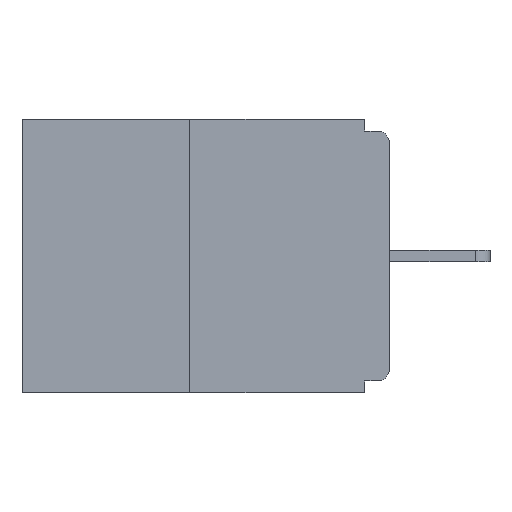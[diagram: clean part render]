
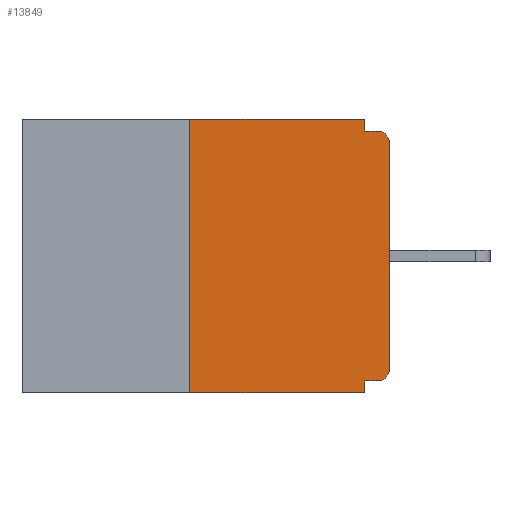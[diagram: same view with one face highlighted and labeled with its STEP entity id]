
A CAD part, left-side view. The second image highlights one B-rep face of the part: STEP entity #13849.
In plain terms, the highlighted planar face has unit normal (-1, 0, 0).
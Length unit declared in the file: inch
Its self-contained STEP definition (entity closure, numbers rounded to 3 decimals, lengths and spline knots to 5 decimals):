
#448 = DIRECTION ( 'NONE',  ( 0., -1., 0. ) ) ;
#521 = VECTOR ( 'NONE', #5096, 39.37008 ) ;
#563 = LINE ( 'NONE', #6883, #10628 ) ;
#835 = DIRECTION ( 'NONE',  ( 0., 0., -1. ) ) ;
#1184 = LINE ( 'NONE', #11006, #7545 ) ;
#1287 = DIRECTION ( 'NONE',  ( 0., -1., 0. ) ) ;
#1321 = VECTOR ( 'NONE', #2225, 39.37008 ) ;
#1588 = CARTESIAN_POINT ( 'NONE',  ( 0., 0.25, 0. ) ) ;
#1994 = CARTESIAN_POINT ( 'NONE',  ( 0., 0.031, 0. ) ) ;
#2058 = ORIENTED_EDGE ( 'NONE', *, *, #6937, .F. ) ;
#2107 = EDGE_CURVE ( 'NONE', #11901, #16938, #563, .T. ) ;
#2209 = ORIENTED_EDGE ( 'NONE', *, *, #16745, .F. ) ;
#2225 = DIRECTION ( 'NONE',  ( 0., 0., 1. ) ) ;
#2241 = CARTESIAN_POINT ( 'NONE',  ( 0., 0.015, -0.313 ) ) ;
#2362 = LINE ( 'NONE', #1994, #7312 ) ;
#2541 = DIRECTION ( 'NONE',  ( -1., 0., 0. ) ) ;
#2736 = VECTOR ( 'NONE', #1287, 39.37008 ) ;
#3031 = DIRECTION ( 'NONE',  ( 0., 0., -1. ) ) ;
#3170 = DIRECTION ( 'NONE',  ( 1., 0., 0. ) ) ;
#3492 = EDGE_CURVE ( 'NONE', #8235, #10366, #2362, .T. ) ;
#3936 = ORIENTED_EDGE ( 'NONE', *, *, #2107, .T. ) ;
#4461 = ORIENTED_EDGE ( 'NONE', *, *, #13895, .F. ) ;
#5003 = CARTESIAN_POINT ( 'NONE',  ( 0., 0.031, -0.015 ) ) ;
#5016 = CARTESIAN_POINT ( 'NONE',  ( 0., 0.031, 0. ) ) ;
#5096 = DIRECTION ( 'NONE',  ( 0., 0., 1. ) ) ;
#5413 = ORIENTED_EDGE ( 'NONE', *, *, #8400, .F. ) ;
#5626 = ORIENTED_EDGE ( 'NONE', *, *, #14633, .T. ) ;
#5666 = DIRECTION ( 'NONE',  ( 0., 1., 0. ) ) ;
#5688 = CARTESIAN_POINT ( 'NONE',  ( 0., 0.015, -0.015 ) ) ;
#5736 = VERTEX_POINT ( 'NONE', #1588 ) ;
#5744 = CARTESIAN_POINT ( 'NONE',  ( 0., 0.25, -0.343 ) ) ;
#6149 = DIRECTION ( 'NONE',  ( 0., 0., -1. ) ) ;
#6883 = CARTESIAN_POINT ( 'NONE',  ( 0., 0.46, -0.343 ) ) ;
#6937 = EDGE_CURVE ( 'NONE', #10366, #11129, #8909, .T. ) ;
#7312 = VECTOR ( 'NONE', #3031, 39.37008 ) ;
#7519 = CARTESIAN_POINT ( 'NONE',  ( 0., 0., -0.03 ) ) ;
#7540 = DIRECTION ( 'NONE',  ( -1., 0., 0. ) ) ;
#7545 = VECTOR ( 'NONE', #5666, 39.37008 ) ;
#7610 = VERTEX_POINT ( 'NONE', #7519 ) ;
#7724 = EDGE_CURVE ( 'NONE', #14753, #7610, #15927, .T. ) ;
#7778 = ORIENTED_EDGE ( 'NONE', *, *, #12898, .F. ) ;
#8079 = VERTEX_POINT ( 'NONE', #16732 ) ;
#8235 = VERTEX_POINT ( 'NONE', #5016 ) ;
#8400 = EDGE_CURVE ( 'NONE', #5736, #8235, #13665, .T. ) ;
#8495 = LINE ( 'NONE', #15901, #9918 ) ;
#8695 = EDGE_CURVE ( 'NONE', #10882, #14753, #8905, .T. ) ;
#8779 = FACE_OUTER_BOUND ( 'NONE', #15231, .T. ) ;
#8905 = CIRCLE ( 'NONE', #13830, 0.015 ) ;
#8909 = LINE ( 'NONE', #11855, #2736 ) ;
#9379 = CIRCLE ( 'NONE', #16709, 0.015 ) ;
#9711 = CARTESIAN_POINT ( 'NONE',  ( 0., 0.46, 0. ) ) ;
#9732 = CARTESIAN_POINT ( 'NONE',  ( 0., 0.46, 0. ) ) ;
#9918 = VECTOR ( 'NONE', #13172, 39.37008 ) ;
#10147 = VECTOR ( 'NONE', #12363, 39.37008 ) ;
#10329 = CARTESIAN_POINT ( 'NONE',  ( 0., 0.25, 0. ) ) ;
#10366 = VERTEX_POINT ( 'NONE', #5003 ) ;
#10628 = VECTOR ( 'NONE', #448, 39.37008 ) ;
#10882 = VERTEX_POINT ( 'NONE', #11561 ) ;
#10945 = PLANE ( 'NONE',  #13310 ) ;
#11006 = CARTESIAN_POINT ( 'NONE',  ( 0., 0., -0.328 ) ) ;
#11059 = DIRECTION ( 'NONE',  ( 0., 0., -1. ) ) ;
#11129 = VERTEX_POINT ( 'NONE', #5688 ) ;
#11561 = CARTESIAN_POINT ( 'NONE',  ( 0., 0.015, -0.328 ) ) ;
#11855 = CARTESIAN_POINT ( 'NONE',  ( 0., 0., -0.015 ) ) ;
#11885 = CARTESIAN_POINT ( 'NONE',  ( 0., 0.031, -0.343 ) ) ;
#11901 = VERTEX_POINT ( 'NONE', #5744 ) ;
#12221 = LINE ( 'NONE', #10329, #1321 ) ;
#12233 = ORIENTED_EDGE ( 'NONE', *, *, #8695, .T. ) ;
#12363 = DIRECTION ( 'NONE',  ( 0., -1., 0. ) ) ;
#12898 = EDGE_CURVE ( 'NONE', #8079, #16938, #8495, .T. ) ;
#13172 = DIRECTION ( 'NONE',  ( 0., 0., -1. ) ) ;
#13310 = AXIS2_PLACEMENT_3D ( 'NONE', #9732, #3170, #11059 ) ;
#13665 = LINE ( 'NONE', #9711, #10147 ) ;
#13830 = AXIS2_PLACEMENT_3D ( 'NONE', #2241, #7540, #835 ) ;
#13849 = ADVANCED_FACE ( 'NONE', ( #8779 ), #10945, .F. ) ;
#13895 = EDGE_CURVE ( 'NONE', #10882, #8079, #1184, .T. ) ;
#14349 = ORIENTED_EDGE ( 'NONE', *, *, #3492, .F. ) ;
#14633 = EDGE_CURVE ( 'NONE', #7610, #11129, #9379, .T. ) ;
#14753 = VERTEX_POINT ( 'NONE', #16831 ) ;
#15005 = ORIENTED_EDGE ( 'NONE', *, *, #7724, .T. ) ;
#15231 = EDGE_LOOP ( 'NONE', ( #5413, #2209, #3936, #7778, #4461, #12233, #15005, #5626, #2058, #14349 ) ) ;
#15817 = CARTESIAN_POINT ( 'NONE',  ( 0., 0.015, -0.03 ) ) ;
#15901 = CARTESIAN_POINT ( 'NONE',  ( 0., 0.031, -0.343 ) ) ;
#15927 = LINE ( 'NONE', #16870, #521 ) ;
#16709 = AXIS2_PLACEMENT_3D ( 'NONE', #15817, #2541, #6149 ) ;
#16732 = CARTESIAN_POINT ( 'NONE',  ( 0., 0.031, -0.328 ) ) ;
#16745 = EDGE_CURVE ( 'NONE', #11901, #5736, #12221, .T. ) ;
#16831 = CARTESIAN_POINT ( 'NONE',  ( 0., 0., -0.313 ) ) ;
#16870 = CARTESIAN_POINT ( 'NONE',  ( 0., 0., 0. ) ) ;
#16938 = VERTEX_POINT ( 'NONE', #11885 ) ;
